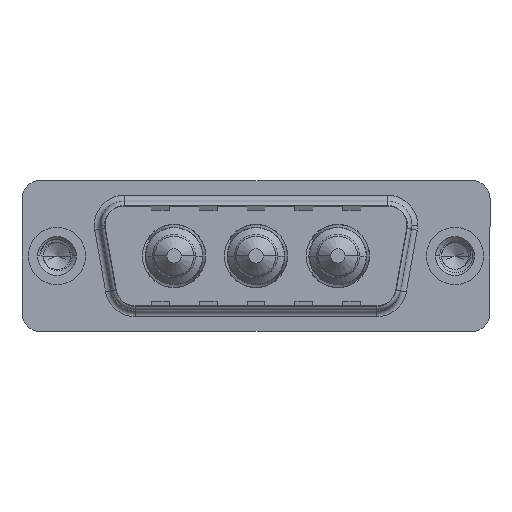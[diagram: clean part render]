
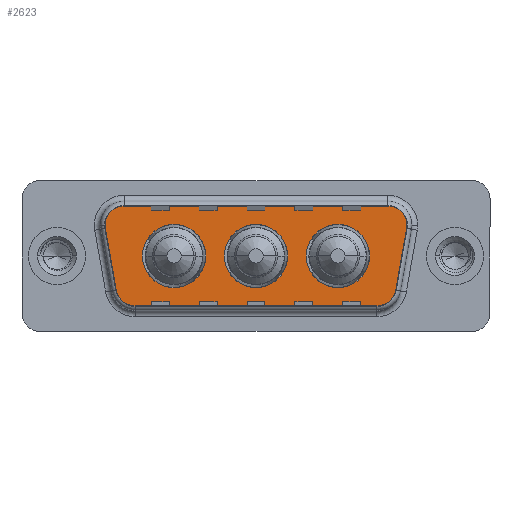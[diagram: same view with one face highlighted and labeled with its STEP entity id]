
A CAD part, top view. The second image highlights one B-rep face of the part: STEP entity #2623.
In plain terms, the highlighted planar face has unit normal (0, 0, 1).
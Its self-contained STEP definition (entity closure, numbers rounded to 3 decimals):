
#17 = VERTEX_POINT ( 'NONE', #10460 ) ;
#72 = DIRECTION ( 'NONE',  ( 1., 0., 0. ) ) ;
#139 = EDGE_CURVE ( 'NONE', #512, #12402, #10514, .T. ) ;
#164 = DIRECTION ( 'NONE',  ( 1., 0., 0. ) ) ;
#232 = AXIS2_PLACEMENT_3D ( 'NONE', #12864, #4370, #14297 ) ;
#235 = CARTESIAN_POINT ( 'NONE',  ( 19.3, 0., 0. ) ) ;
#291 = ORIENTED_EDGE ( 'NONE', *, *, #15458, .T. ) ;
#512 = VERTEX_POINT ( 'NONE', #9345 ) ;
#685 = FACE_BOUND ( 'NONE', #1794, .T. ) ;
#849 = CARTESIAN_POINT ( 'NONE',  ( 20.85, 0., 0. ) ) ;
#1152 = CARTESIAN_POINT ( 'NONE',  ( 28.836, -3.247, 0. ) ) ;
#1341 = LINE ( 'NONE', #1516, #7899 ) ;
#1363 = ORIENTED_EDGE ( 'NONE', *, *, #11141, .T. ) ;
#1437 = AXIS2_PLACEMENT_3D ( 'NONE', #13575, #13641, #6139 ) ;
#1516 = CARTESIAN_POINT ( 'NONE',  ( 6.434, -4.9, 0. ) ) ;
#1585 = VERTEX_POINT ( 'NONE', #2235 ) ;
#1794 = EDGE_LOOP ( 'NONE', ( #15196, #12149 ) ) ;
#1853 = LINE ( 'NONE', #11096, #8848 ) ;
#1881 = DIRECTION ( 'NONE',  ( 0., 0., 1. ) ) ;
#1946 = ORIENTED_EDGE ( 'NONE', *, *, #3990, .F. ) ;
#2111 = EDGE_LOOP ( 'NONE', ( #1946, #8604 ) ) ;
#2235 = CARTESIAN_POINT ( 'NONE',  ( 5.411, 4.9, 0. ) ) ;
#2275 = CARTESIAN_POINT ( 'NONE',  ( 5.411, 4.9, 0. ) ) ;
#2313 = CIRCLE ( 'NONE', #3634, 2.65 ) ;
#2623 = ADVANCED_FACE ( 'NONE', ( #7636, #685, #15139, #3869 ), #3682, .T. ) ;
#2647 = CARTESIAN_POINT ( 'NONE',  ( 27.889, 2.9, 0. ) ) ;
#2727 = EDGE_CURVE ( 'NONE', #8974, #2817, #13835, .T. ) ;
#2790 = EDGE_CURVE ( 'NONE', #17, #8337, #9616, .T. ) ;
#2817 = VERTEX_POINT ( 'NONE', #13945 ) ;
#3604 = CARTESIAN_POINT ( 'NONE',  ( 23.5, 0., 0. ) ) ;
#3634 = AXIS2_PLACEMENT_3D ( 'NONE', #14128, #5600, #15475 ) ;
#3682 = PLANE ( 'NONE',  #9298 ) ;
#3700 = ORIENTED_EDGE ( 'NONE', *, *, #2790, .T. ) ;
#3803 = DIRECTION ( 'NONE',  ( 0., 0., 1. ) ) ;
#3869 = FACE_OUTER_BOUND ( 'NONE', #5203, .T. ) ;
#3907 = DIRECTION ( 'NONE',  ( 1., 0., 0. ) ) ;
#3990 = EDGE_CURVE ( 'NONE', #9555, #5683, #14050, .T. ) ;
#3997 = DIRECTION ( 'NONE',  ( -1., 0., 0. ) ) ;
#4022 = EDGE_LOOP ( 'NONE', ( #17042, #13276 ) ) ;
#4137 = CARTESIAN_POINT ( 'NONE',  ( 3.441, 2.553, 0. ) ) ;
#4159 = CIRCLE ( 'NONE', #13488, 2.65 ) ;
#4288 = DIRECTION ( 'NONE',  ( 0., 0., 1. ) ) ;
#4370 = DIRECTION ( 'NONE',  ( 0., 0., 1. ) ) ;
#4504 = DIRECTION ( 'NONE',  ( 0., 0., 1. ) ) ;
#4663 = DIRECTION ( 'NONE',  ( 0.174, -0.985, 0. ) ) ;
#5012 = DIRECTION ( 'NONE',  ( 1., 0., 0. ) ) ;
#5024 = CARTESIAN_POINT ( 'NONE',  ( 14., 0., 0. ) ) ;
#5082 = AXIS2_PLACEMENT_3D ( 'NONE', #12778, #4288, #14221 ) ;
#5203 = EDGE_LOOP ( 'NONE', ( #3700, #16680, #6687, #9955, #14494, #15541, #11705, #1363, #291 ) ) ;
#5600 = DIRECTION ( 'NONE',  ( 0., 0., 1. ) ) ;
#5683 = VERTEX_POINT ( 'NONE', #5024 ) ;
#6095 = CARTESIAN_POINT ( 'NONE',  ( 12.45, 0., 0. ) ) ;
#6139 = DIRECTION ( 'NONE',  ( 1., 0., 0. ) ) ;
#6168 = CARTESIAN_POINT ( 'NONE',  ( 27.889, 4.9, 0. ) ) ;
#6408 = CIRCLE ( 'NONE', #7077, 2. ) ;
#6429 = VERTEX_POINT ( 'NONE', #849 ) ;
#6687 = ORIENTED_EDGE ( 'NONE', *, *, #2727, .T. ) ;
#6689 = CARTESIAN_POINT ( 'NONE',  ( 27.889, 2.9, 0. ) ) ;
#6743 = VECTOR ( 'NONE', #4663, 1000. ) ;
#7054 = VERTEX_POINT ( 'NONE', #16082 ) ;
#7077 = AXIS2_PLACEMENT_3D ( 'NONE', #16595, #8318, #17888 ) ;
#7080 = DIRECTION ( 'NONE',  ( 0., 0., 1. ) ) ;
#7275 = EDGE_CURVE ( 'NONE', #17304, #7054, #2313, .T. ) ;
#7473 = CARTESIAN_POINT ( 'NONE',  ( 16.65, 0., 0. ) ) ;
#7498 = DIRECTION ( 'NONE',  ( -1., 0., 0. ) ) ;
#7636 = FACE_BOUND ( 'NONE', #2111, .T. ) ;
#7899 = VECTOR ( 'NONE', #164, 1000. ) ;
#8318 = DIRECTION ( 'NONE',  ( 0., 0., 1. ) ) ;
#8337 = VERTEX_POINT ( 'NONE', #1152 ) ;
#8456 = EDGE_CURVE ( 'NONE', #8337, #8974, #1853, .T. ) ;
#8516 = EDGE_CURVE ( 'NONE', #14100, #6429, #13033, .T. ) ;
#8531 = EDGE_CURVE ( 'NONE', #14885, #1585, #11707, .T. ) ;
#8581 = EDGE_CURVE ( 'NONE', #6429, #14100, #4159, .T. ) ;
#8604 = ORIENTED_EDGE ( 'NONE', *, *, #11922, .F. ) ;
#8848 = VECTOR ( 'NONE', #15327, 1000. ) ;
#8974 = VERTEX_POINT ( 'NONE', #10840 ) ;
#9298 = AXIS2_PLACEMENT_3D ( 'NONE', #12993, #11439, #3907 ) ;
#9345 = CARTESIAN_POINT ( 'NONE',  ( 3.441, 2.553, 0. ) ) ;
#9548 = CARTESIAN_POINT ( 'NONE',  ( 6.434, -4.9, 0. ) ) ;
#9555 = VERTEX_POINT ( 'NONE', #235 ) ;
#9616 = CIRCLE ( 'NONE', #1437, 2. ) ;
#9955 = ORIENTED_EDGE ( 'NONE', *, *, #16965, .T. ) ;
#10243 = CARTESIAN_POINT ( 'NONE',  ( 5.411, 2.9, 0. ) ) ;
#10460 = CARTESIAN_POINT ( 'NONE',  ( 26.866, -4.9, 0. ) ) ;
#10514 = LINE ( 'NONE', #4137, #6743 ) ;
#10633 = AXIS2_PLACEMENT_3D ( 'NONE', #3604, #13511, #5012 ) ;
#10650 = DIRECTION ( 'NONE',  ( -1., 0., 0. ) ) ;
#10840 = CARTESIAN_POINT ( 'NONE',  ( 29.859, 2.553, 0. ) ) ;
#11096 = CARTESIAN_POINT ( 'NONE',  ( 29.859, 2.553, 0. ) ) ;
#11141 = EDGE_CURVE ( 'NONE', #12402, #16188, #6408, .T. ) ;
#11259 = VECTOR ( 'NONE', #10650, 1000. ) ;
#11268 = EDGE_CURVE ( 'NONE', #7054, #17304, #15423, .T. ) ;
#11301 = AXIS2_PLACEMENT_3D ( 'NONE', #7473, #3803, #72 ) ;
#11439 = DIRECTION ( 'NONE',  ( 0., 0., 1. ) ) ;
#11678 = DIRECTION ( 'NONE',  ( 1., 0., 0. ) ) ;
#11705 = ORIENTED_EDGE ( 'NONE', *, *, #139, .T. ) ;
#11707 = LINE ( 'NONE', #2275, #11259 ) ;
#11922 = EDGE_CURVE ( 'NONE', #5683, #9555, #15014, .T. ) ;
#12031 = EDGE_CURVE ( 'NONE', #1585, #512, #13239, .T. ) ;
#12149 = ORIENTED_EDGE ( 'NONE', *, *, #8581, .F. ) ;
#12402 = VERTEX_POINT ( 'NONE', #16432 ) ;
#12473 = DIRECTION ( 'NONE',  ( 0., 0., 1. ) ) ;
#12778 = CARTESIAN_POINT ( 'NONE',  ( 16.65, 0., 0. ) ) ;
#12864 = CARTESIAN_POINT ( 'NONE',  ( 9.8, 0., 0. ) ) ;
#12993 = CARTESIAN_POINT ( 'NONE',  ( 26.866, -2.9, 0. ) ) ;
#13033 = CIRCLE ( 'NONE', #10633, 2.65 ) ;
#13239 = CIRCLE ( 'NONE', #17202, 2. ) ;
#13276 = ORIENTED_EDGE ( 'NONE', *, *, #11268, .F. ) ;
#13488 = AXIS2_PLACEMENT_3D ( 'NONE', #15515, #7080, #16804 ) ;
#13511 = DIRECTION ( 'NONE',  ( 0., 0., 1. ) ) ;
#13575 = CARTESIAN_POINT ( 'NONE',  ( 26.866, -2.9, 0. ) ) ;
#13641 = DIRECTION ( 'NONE',  ( 0., 0., 1. ) ) ;
#13835 = CIRCLE ( 'NONE', #14010, 2. ) ;
#13945 = CARTESIAN_POINT ( 'NONE',  ( 29.889, 2.9, 0. ) ) ;
#14010 = AXIS2_PLACEMENT_3D ( 'NONE', #6689, #4504, #7498 ) ;
#14050 = CIRCLE ( 'NONE', #11301, 2.65 ) ;
#14100 = VERTEX_POINT ( 'NONE', #17803 ) ;
#14128 = CARTESIAN_POINT ( 'NONE',  ( 9.8, 0., 0. ) ) ;
#14221 = DIRECTION ( 'NONE',  ( 1., 0., 0. ) ) ;
#14297 = DIRECTION ( 'NONE',  ( 1., 0., 0. ) ) ;
#14494 = ORIENTED_EDGE ( 'NONE', *, *, #8531, .T. ) ;
#14885 = VERTEX_POINT ( 'NONE', #6168 ) ;
#15014 = CIRCLE ( 'NONE', #5082, 2.65 ) ;
#15139 = FACE_BOUND ( 'NONE', #4022, .T. ) ;
#15196 = ORIENTED_EDGE ( 'NONE', *, *, #8516, .F. ) ;
#15327 = DIRECTION ( 'NONE',  ( 0.174, 0.985, 0. ) ) ;
#15423 = CIRCLE ( 'NONE', #232, 2.65 ) ;
#15458 = EDGE_CURVE ( 'NONE', #16188, #17, #1341, .T. ) ;
#15475 = DIRECTION ( 'NONE',  ( 1., 0., 0. ) ) ;
#15515 = CARTESIAN_POINT ( 'NONE',  ( 23.5, 0., 0. ) ) ;
#15541 = ORIENTED_EDGE ( 'NONE', *, *, #12031, .T. ) ;
#16082 = CARTESIAN_POINT ( 'NONE',  ( 7.15, 0., 0. ) ) ;
#16188 = VERTEX_POINT ( 'NONE', #9548 ) ;
#16304 = CIRCLE ( 'NONE', #17479, 2. ) ;
#16432 = CARTESIAN_POINT ( 'NONE',  ( 4.464, -3.247, 0. ) ) ;
#16595 = CARTESIAN_POINT ( 'NONE',  ( 6.434, -2.9, 0. ) ) ;
#16680 = ORIENTED_EDGE ( 'NONE', *, *, #8456, .T. ) ;
#16804 = DIRECTION ( 'NONE',  ( 1., 0., 0. ) ) ;
#16965 = EDGE_CURVE ( 'NONE', #2817, #14885, #16304, .T. ) ;
#17042 = ORIENTED_EDGE ( 'NONE', *, *, #7275, .F. ) ;
#17202 = AXIS2_PLACEMENT_3D ( 'NONE', #10243, #1881, #11678 ) ;
#17304 = VERTEX_POINT ( 'NONE', #6095 ) ;
#17479 = AXIS2_PLACEMENT_3D ( 'NONE', #2647, #12473, #3997 ) ;
#17803 = CARTESIAN_POINT ( 'NONE',  ( 26.15, 0., 0. ) ) ;
#17888 = DIRECTION ( 'NONE',  ( -1., 0., 0. ) ) ;
